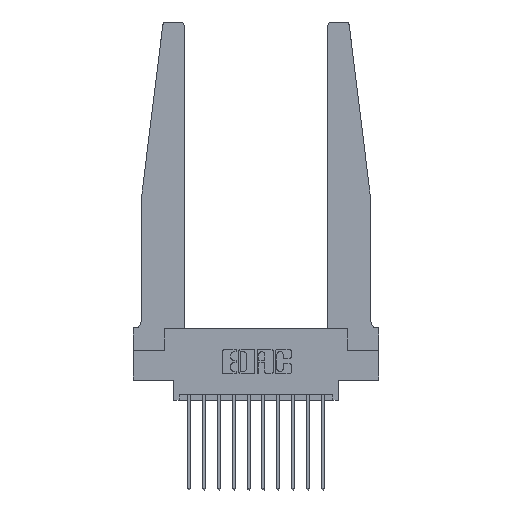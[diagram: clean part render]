
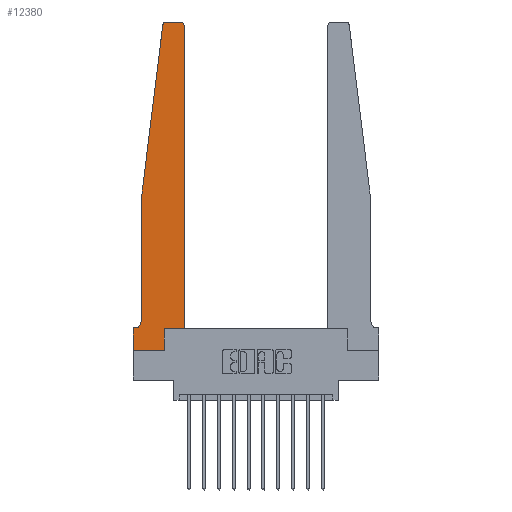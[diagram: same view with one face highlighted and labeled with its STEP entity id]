
A CAD part, top view. The second image highlights one B-rep face of the part: STEP entity #12380.
In plain terms, the highlighted planar face has unit normal (0, 0, 1).
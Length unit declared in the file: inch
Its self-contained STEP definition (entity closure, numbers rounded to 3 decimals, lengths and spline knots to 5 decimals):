
#100 = DIRECTION ( 'NONE',  ( 0., 0., 1. ) ) ;
#122 = EDGE_CURVE ( 'NONE', #14627, #13179, #13344, .T. ) ;
#856 = CARTESIAN_POINT ( 'NONE',  ( 0.25, 2.75, 0.37 ) ) ;
#935 = CARTESIAN_POINT ( 'NONE',  ( 0.27653, 2.72, 0.37 ) ) ;
#1197 = AXIS2_PLACEMENT_3D ( 'NONE', #12873, #9102, #6730 ) ;
#1254 = EDGE_CURVE ( 'NONE', #13179, #8487, #8456, .T. ) ;
#1444 = ORIENTED_EDGE ( 'NONE', *, *, #15568, .T. ) ;
#1766 = VECTOR ( 'NONE', #11769, 39.37008 ) ;
#1809 = LINE ( 'NONE', #12927, #1766 ) ;
#1856 = EDGE_CURVE ( 'NONE', #7587, #6759, #2315, .T. ) ;
#1978 = ORIENTED_EDGE ( 'NONE', *, *, #3157, .T. ) ;
#2315 = LINE ( 'NONE', #11211, #14121 ) ;
#2390 = DIRECTION ( 'NONE',  ( 0., 1., 0. ) ) ;
#2420 = DIRECTION ( 'NONE',  ( 1., 0., 0. ) ) ;
#2524 = CARTESIAN_POINT ( 'NONE',  ( 0., 0.1875, 0.37 ) ) ;
#2547 = CARTESIAN_POINT ( 'NONE',  ( 0.395, 2.75, 0.37 ) ) ;
#3157 = EDGE_CURVE ( 'NONE', #10962, #8153, #4926, .T. ) ;
#3213 = LINE ( 'NONE', #7359, #5905 ) ;
#3215 = CARTESIAN_POINT ( 'NONE',  ( 0.065, 1.25, 0.37 ) ) ;
#3444 = DIRECTION ( 'NONE',  ( 0., 1., 0. ) ) ;
#3479 = DIRECTION ( 'NONE',  ( 1., 0., 0. ) ) ;
#3744 = DIRECTION ( 'NONE',  ( 0., 0., 1. ) ) ;
#3875 = VERTEX_POINT ( 'NONE', #11650 ) ;
#4039 = ORIENTED_EDGE ( 'NONE', *, *, #15433, .T. ) ;
#4057 = PLANE ( 'NONE',  #11081 ) ;
#4097 = CARTESIAN_POINT ( 'NONE',  ( 0., 0., 0.37 ) ) ;
#4349 = ORIENTED_EDGE ( 'NONE', *, *, #15364, .T. ) ;
#4371 = DIRECTION ( 'NONE',  ( 1., 0., 0. ) ) ;
#4389 = VERTEX_POINT ( 'NONE', #10709 ) ;
#4503 = EDGE_CURVE ( 'NONE', #3875, #14894, #15953, .T. ) ;
#4544 = DIRECTION ( 'NONE',  ( -1., 0., 0. ) ) ;
#4611 = VECTOR ( 'NONE', #3479, 39.37008 ) ;
#4701 = CARTESIAN_POINT ( 'NONE',  ( 0.425, 0.18, 0.37 ) ) ;
#4926 = LINE ( 'NONE', #4097, #6574 ) ;
#5397 = DIRECTION ( 'NONE',  ( 0., -1., 0. ) ) ;
#5905 = VECTOR ( 'NONE', #2390, 39.37008 ) ;
#5919 = DIRECTION ( 'NONE',  ( 0., 0., 1. ) ) ;
#6288 = CARTESIAN_POINT ( 'NONE',  ( 0.065, 1.25, 0.37 ) ) ;
#6574 = VECTOR ( 'NONE', #5397, 39.37008 ) ;
#6730 = DIRECTION ( 'NONE',  ( -1., 0., 0. ) ) ;
#6755 = ORIENTED_EDGE ( 'NONE', *, *, #4503, .T. ) ;
#6759 = VERTEX_POINT ( 'NONE', #7790 ) ;
#6816 = CARTESIAN_POINT ( 'NONE',  ( 0.24675, 2.72367, 0.37 ) ) ;
#6834 = CARTESIAN_POINT ( 'NONE',  ( 0.2605, 0.18, 0.37 ) ) ;
#6845 = CARTESIAN_POINT ( 'NONE',  ( 0., 0., 0.37 ) ) ;
#6906 = CARTESIAN_POINT ( 'NONE',  ( 0.015, 0.1875, 0.37 ) ) ;
#6963 = DIRECTION ( 'NONE',  ( -0.122, -0.992, 0. ) ) ;
#7359 = CARTESIAN_POINT ( 'NONE',  ( 0.425, 0.18, 0.37 ) ) ;
#7516 = CARTESIAN_POINT ( 'NONE',  ( 0., 0.1875, 0.37 ) ) ;
#7556 = AXIS2_PLACEMENT_3D ( 'NONE', #7619, #100, #11591 ) ;
#7587 = VERTEX_POINT ( 'NONE', #6288 ) ;
#7619 = CARTESIAN_POINT ( 'NONE',  ( 0.395, 2.72, 0.37 ) ) ;
#7790 = CARTESIAN_POINT ( 'NONE',  ( 0.065, 0.2375, 0.37 ) ) ;
#7817 = EDGE_CURVE ( 'NONE', #8672, #10962, #1809, .T. ) ;
#8153 = VERTEX_POINT ( 'NONE', #6845 ) ;
#8456 = LINE ( 'NONE', #856, #15008 ) ;
#8487 = VERTEX_POINT ( 'NONE', #12886 ) ;
#8672 = VERTEX_POINT ( 'NONE', #6906 ) ;
#9102 = DIRECTION ( 'NONE',  ( 0., 0., -1. ) ) ;
#9302 = AXIS2_PLACEMENT_3D ( 'NONE', #935, #5919, #2420 ) ;
#9597 = VECTOR ( 'NONE', #3444, 39.37008 ) ;
#9644 = CARTESIAN_POINT ( 'NONE',  ( 0.2605, 0.18, 0.37 ) ) ;
#9793 = CIRCLE ( 'NONE', #1197, 0.05 ) ;
#9917 = ORIENTED_EDGE ( 'NONE', *, *, #7817, .T. ) ;
#10709 = CARTESIAN_POINT ( 'NONE',  ( 0.425, 0.18, 0.37 ) ) ;
#10848 = ORIENTED_EDGE ( 'NONE', *, *, #1254, .T. ) ;
#10962 = VERTEX_POINT ( 'NONE', #7516 ) ;
#11081 = AXIS2_PLACEMENT_3D ( 'NONE', #2524, #3744, #12562 ) ;
#11121 = ORIENTED_EDGE ( 'NONE', *, *, #1856, .T. ) ;
#11127 = DIRECTION ( 'NONE',  ( 0., -1., 0. ) ) ;
#11211 = CARTESIAN_POINT ( 'NONE',  ( 0.065, 1.25, 0.37 ) ) ;
#11412 = FACE_OUTER_BOUND ( 'NONE', #15998, .T. ) ;
#11591 = DIRECTION ( 'NONE',  ( 1., 0., 0. ) ) ;
#11650 = CARTESIAN_POINT ( 'NONE',  ( 0.2605, 0., 0.37 ) ) ;
#11704 = LINE ( 'NONE', #3215, #14291 ) ;
#11769 = DIRECTION ( 'NONE',  ( -1., 0., 0. ) ) ;
#11781 = ORIENTED_EDGE ( 'NONE', *, *, #14821, .T. ) ;
#12347 = ORIENTED_EDGE ( 'NONE', *, *, #122, .T. ) ;
#12368 = LINE ( 'NONE', #4701, #4611 ) ;
#12380 = ADVANCED_FACE ( 'NONE', ( #11412 ), #4057, .T. ) ;
#12562 = DIRECTION ( 'NONE',  ( 1., 0., 0. ) ) ;
#12873 = CARTESIAN_POINT ( 'NONE',  ( 0.015, 0.2375, 0.37 ) ) ;
#12886 = CARTESIAN_POINT ( 'NONE',  ( 0.27653, 2.75, 0.37 ) ) ;
#12927 = CARTESIAN_POINT ( 'NONE',  ( 0.065, 0.1875, 0.37 ) ) ;
#13136 = ORIENTED_EDGE ( 'NONE', *, *, #14164, .T. ) ;
#13178 = ORIENTED_EDGE ( 'NONE', *, *, #15225, .T. ) ;
#13179 = VERTEX_POINT ( 'NONE', #2547 ) ;
#13233 = VECTOR ( 'NONE', #4371, 39.37008 ) ;
#13344 = CIRCLE ( 'NONE', #7556, 0.03 ) ;
#14121 = VECTOR ( 'NONE', #11127, 39.37008 ) ;
#14159 = VERTEX_POINT ( 'NONE', #6816 ) ;
#14164 = EDGE_CURVE ( 'NONE', #6759, #8672, #9793, .T. ) ;
#14281 = CIRCLE ( 'NONE', #9302, 0.03 ) ;
#14291 = VECTOR ( 'NONE', #6963, 39.37008 ) ;
#14489 = CARTESIAN_POINT ( 'NONE',  ( 0.425, 2.72, 0.37 ) ) ;
#14627 = VERTEX_POINT ( 'NONE', #14489 ) ;
#14821 = EDGE_CURVE ( 'NONE', #4389, #14627, #3213, .T. ) ;
#14894 = VERTEX_POINT ( 'NONE', #6834 ) ;
#15008 = VECTOR ( 'NONE', #4544, 39.37008 ) ;
#15225 = EDGE_CURVE ( 'NONE', #8153, #3875, #15510, .T. ) ;
#15364 = EDGE_CURVE ( 'NONE', #14894, #4389, #12368, .T. ) ;
#15433 = EDGE_CURVE ( 'NONE', #8487, #14159, #14281, .T. ) ;
#15510 = LINE ( 'NONE', #15681, #13233 ) ;
#15568 = EDGE_CURVE ( 'NONE', #14159, #7587, #11704, .T. ) ;
#15681 = CARTESIAN_POINT ( 'NONE',  ( 0., 0., 0.37 ) ) ;
#15953 = LINE ( 'NONE', #9644, #9597 ) ;
#15998 = EDGE_LOOP ( 'NONE', ( #10848, #4039, #1444, #11121, #13136, #9917, #1978, #13178, #6755, #4349, #11781, #12347 ) ) ;
